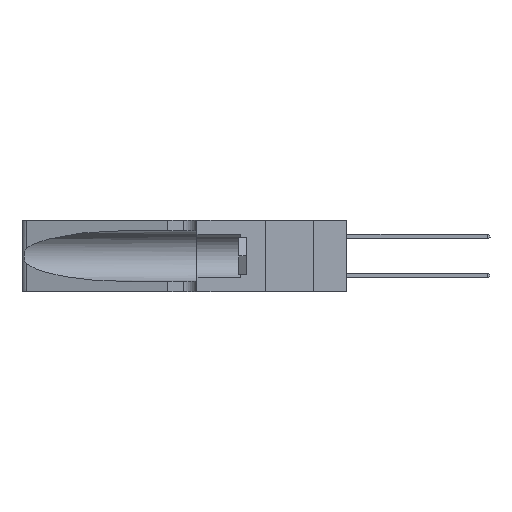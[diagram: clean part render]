
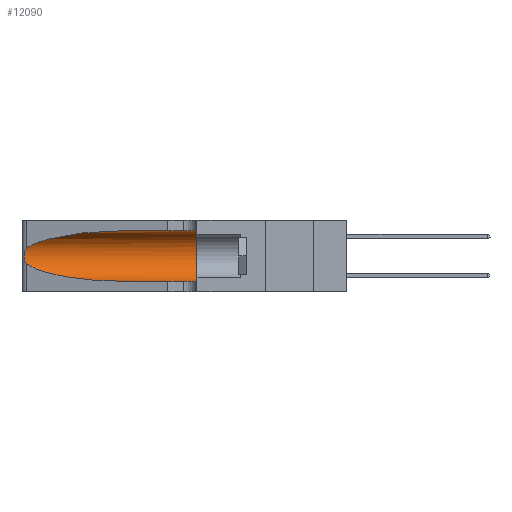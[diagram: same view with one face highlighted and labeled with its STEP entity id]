
A CAD part, left-side view. The second image highlights one B-rep face of the part: STEP entity #12090.
In plain terms, the highlighted cylindrical face has radius 3.308 mm (diameter 6.617 mm), a partial arc.
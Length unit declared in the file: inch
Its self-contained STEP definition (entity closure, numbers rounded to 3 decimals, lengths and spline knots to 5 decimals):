
#283 = CARTESIAN_POINT ( 'NONE',  ( 0.26075, 1.23896, 0.19203 ) ) ;
#327 = EDGE_LOOP ( 'NONE', ( #27973, #27629, #20958, #22075, #3037, #888 ) ) ;
#888 = ORIENTED_EDGE ( 'NONE', *, *, #13011, .F. ) ;
#1913 = VERTEX_POINT ( 'NONE', #27180 ) ;
#2774 = CARTESIAN_POINT ( 'NONE',  ( 0.1305, 0.72297, 0.31525 ) ) ;
#3037 = ORIENTED_EDGE ( 'NONE', *, *, #43421, .F. ) ;
#3754 = CARTESIAN_POINT ( 'NONE',  ( 0.25487, 1.22718, 0.14631 ) ) ;
#3887 = CARTESIAN_POINT ( 'NONE',  ( 0.26017, 1.23833, 0.17102 ) ) ;
#5836 = VERTEX_POINT ( 'NONE', #12551 ) ;
#6670 = DIRECTION ( 'NONE',  ( 0., 1., 0. ) ) ;
#7325 = CARTESIAN_POINT ( 'NONE',  ( 0.18966, 0.96281, 0.05475 ) ) ;
#7464 = CARTESIAN_POINT ( 'NONE',  ( 0.25789, 1.23486, 0.15765 ) ) ;
#9549 = VERTEX_POINT ( 'NONE', #17150 ) ;
#10708 = DIRECTION ( 'NONE',  ( 0., -1., 0. ) ) ;
#10865 = CARTESIAN_POINT ( 'NONE',  ( 0.25487, 1.22718, 0.22369 ) ) ;
#11014 = CARTESIAN_POINT ( 'NONE',  ( 0.25555, 1.22993, 0.14849 ) ) ;
#12090 = ADVANCED_FACE ( 'NONE', ( #32886 ), #22712, .F. ) ;
#12551 = CARTESIAN_POINT ( 'NONE',  ( 0.25487, 1.22718, 0.22369 ) ) ;
#13011 = EDGE_CURVE ( 'NONE', #32565, #41121, #41470, .T. ) ;
#13481 = CARTESIAN_POINT ( 'NONE',  ( 0.2373, 1.15595, 0.28018 ) ) ;
#13852 = VECTOR ( 'NONE', #28942, 39.37008 ) ;
#15194 = CARTESIAN_POINT ( 'NONE',  ( 0.1305, 1.61858, 0.05475 ) ) ;
#16752 = B_SPLINE_CURVE_WITH_KNOTS ( 'NONE', 3,
 ( #10865, #31496, #38397, #17901, #41827, #21309, #283, #24742, #3887, #28196, #7464, #31638, #11014, #35074 ),
 .UNSPECIFIED., .F., .F.,
 ( 4, 2, 2, 2, 2, 2, 4 ),
 ( 0., 0.00027, 0.00053, 0.00107, 0.0016, 0.00187, 0.00214 ),
 .UNSPECIFIED. ) ;
#17150 = CARTESIAN_POINT ( 'NONE',  ( 0.1305, 0.35, 0.05475 ) ) ;
#17901 = CARTESIAN_POINT ( 'NONE',  ( 0.25787, 1.23484, 0.2124 ) ) ;
#19017 = DIRECTION ( 'NONE',  ( 0., -1., 0. ) ) ;
#20958 = ORIENTED_EDGE ( 'NONE', *, *, #35445, .T. ) ;
#21309 = CARTESIAN_POINT ( 'NONE',  ( 0.26018, 1.23835, 0.19895 ) ) ;
#22061 = CARTESIAN_POINT ( 'NONE',  ( 0.1305, 0.35, 0.31525 ) ) ;
#22075 = ORIENTED_EDGE ( 'NONE', *, *, #35584, .T. ) ;
#22712 = CYLINDRICAL_SURFACE ( 'NONE', #38287, 0.13025 ) ;
#22969 = LINE ( 'NONE', #15194, #13852 ) ;
#23168 = CARTESIAN_POINT ( 'NONE',  ( 0.25487, 1.22718, 0.14631 ) ) ;
#24612 = CARTESIAN_POINT ( 'NONE',  ( 0.2373, 1.15595, 0.08982 ) ) ;
#24742 = CARTESIAN_POINT ( 'NONE',  ( 0.26075, 1.23896, 0.178 ) ) ;
#27180 = CARTESIAN_POINT ( 'NONE',  ( 0.1305, 0.72297, 0.05475 ) ) ;
#27454 = CARTESIAN_POINT ( 'NONE',  ( 0.1305, 0.35, 0.185 ) ) ;
#27629 = ORIENTED_EDGE ( 'NONE', *, *, #44121, .T. ) ;
#27900 = CARTESIAN_POINT ( 'NONE',  ( 0.1305, 1.61858, 0.185 ) ) ;
#27973 = ORIENTED_EDGE ( 'NONE', *, *, #35915, .T. ) ;
#28196 = CARTESIAN_POINT ( 'NONE',  ( 0.25856, 1.23593, 0.16098 ) ) ;
#28942 = DIRECTION ( 'NONE',  ( 0., -1., 0. ) ) ;
#29158 = CARTESIAN_POINT ( 'NONE',  ( 0.1305, 1.61858, 0.31525 ) ) ;
#30583 = CARTESIAN_POINT ( 'NONE',  ( 0.18966, 0.96281, 0.31525 ) ) ;
#30891 = DIRECTION ( 'NONE',  ( 0., 0., 1. ) ) ;
#31496 = CARTESIAN_POINT ( 'NONE',  ( 0.25555, 1.22994, 0.2215 ) ) ;
#31510 = CARTESIAN_POINT ( 'NONE',  ( 0.1305, 0.72297, 0.05475 ) ) ;
#31638 = CARTESIAN_POINT ( 'NONE',  ( 0.25639, 1.23186, 0.15144 ) ) ;
#32336 = VECTOR ( 'NONE', #19017, 39.37008 ) ;
#32565 = VERTEX_POINT ( 'NONE', #37872 ) ;
#32620 =( BOUNDED_CURVE ( )  B_SPLINE_CURVE ( 3, ( #2774, #30583, #13481, #37481 ),
 .UNSPECIFIED., .F., .F. ) 
 B_SPLINE_CURVE_WITH_KNOTS ( ( 4, 4 ),
 ( 1.5708, 2.84003 ),
 .UNSPECIFIED. ) 
 CURVE ( )  GEOMETRIC_REPRESENTATION_ITEM ( )  RATIONAL_B_SPLINE_CURVE ( ( 1., 0.87, 0.87, 1. ) ) 
 REPRESENTATION_ITEM ( '' )  );
#32886 = FACE_OUTER_BOUND ( 'NONE', #327, .T. ) ;
#34760 = DIRECTION ( 'NONE',  ( 0., 0., -1. ) ) ;
#35074 = CARTESIAN_POINT ( 'NONE',  ( 0.25487, 1.22718, 0.14631 ) ) ;
#35445 = EDGE_CURVE ( 'NONE', #37066, #1913, #40616, .T. ) ;
#35584 = EDGE_CURVE ( 'NONE', #1913, #9549, #22969, .T. ) ;
#35915 = EDGE_CURVE ( 'NONE', #32565, #5836, #32620, .T. ) ;
#37066 = VERTEX_POINT ( 'NONE', #23168 ) ;
#37338 = AXIS2_PLACEMENT_3D ( 'NONE', #27454, #6670, #30891 ) ;
#37481 = CARTESIAN_POINT ( 'NONE',  ( 0.25487, 1.22718, 0.22369 ) ) ;
#37872 = CARTESIAN_POINT ( 'NONE',  ( 0.1305, 0.72297, 0.31525 ) ) ;
#38287 = AXIS2_PLACEMENT_3D ( 'NONE', #27900, #10708, #34760 ) ;
#38397 = CARTESIAN_POINT ( 'NONE',  ( 0.25639, 1.23184, 0.21858 ) ) ;
#40616 =( BOUNDED_CURVE ( )  B_SPLINE_CURVE ( 3, ( #3754, #24612, #7325, #31510 ),
 .UNSPECIFIED., .F., .T. ) 
 B_SPLINE_CURVE_WITH_KNOTS ( ( 4, 4 ),
 ( 3.44316, 4.71239 ),
 .UNSPECIFIED. ) 
 CURVE ( )  GEOMETRIC_REPRESENTATION_ITEM ( )  RATIONAL_B_SPLINE_CURVE ( ( 1., 0.87, 0.87, 1. ) ) 
 REPRESENTATION_ITEM ( '' )  );
#41121 = VERTEX_POINT ( 'NONE', #22061 ) ;
#41470 = LINE ( 'NONE', #29158, #32336 ) ;
#41827 = CARTESIAN_POINT ( 'NONE',  ( 0.25854, 1.2359, 0.20912 ) ) ;
#43421 = EDGE_CURVE ( 'NONE', #41121, #9549, #43767, .T. ) ;
#43767 = CIRCLE ( 'NONE', #37338, 0.13025 ) ;
#44121 = EDGE_CURVE ( 'NONE', #5836, #37066, #16752, .T. ) ;
